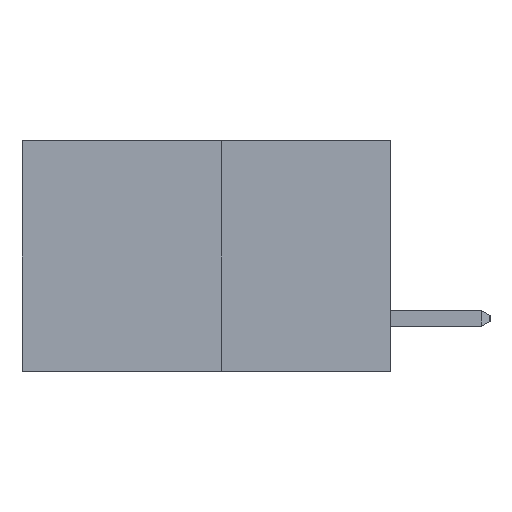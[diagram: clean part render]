
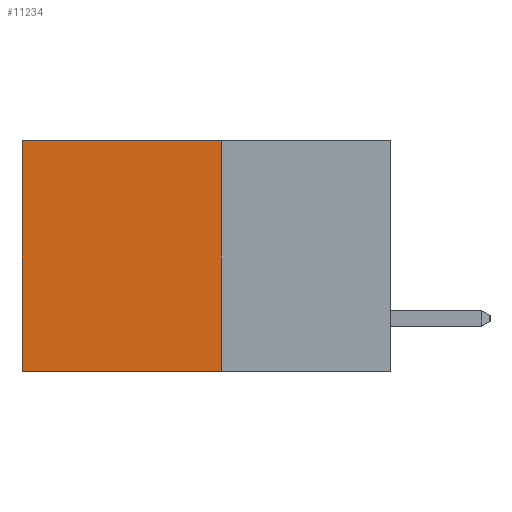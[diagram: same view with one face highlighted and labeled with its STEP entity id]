
A CAD part, left-side view. The second image highlights one B-rep face of the part: STEP entity #11234.
In plain terms, the highlighted planar face has unit normal (-1, 0, 0).
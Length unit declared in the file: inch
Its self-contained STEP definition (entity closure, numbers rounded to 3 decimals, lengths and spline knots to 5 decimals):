
#437 = EDGE_LOOP ( 'NONE', ( #1618, #18572, #18990, #6859 ) ) ;
#762 = DIRECTION ( 'NONE',  ( 0., 0., -1. ) ) ;
#764 = EDGE_CURVE ( 'NONE', #14618, #11002, #4069, .T. ) ;
#1229 = LINE ( 'NONE', #17174, #17666 ) ;
#1618 = ORIENTED_EDGE ( 'NONE', *, *, #764, .T. ) ;
#2950 = VERTEX_POINT ( 'NONE', #10040 ) ;
#3100 = EDGE_CURVE ( 'NONE', #2950, #14618, #7274, .T. ) ;
#3221 = VECTOR ( 'NONE', #16580, 39.37008 ) ;
#4069 = LINE ( 'NONE', #8759, #12252 ) ;
#4211 = AXIS2_PLACEMENT_3D ( 'NONE', #4647, #17748, #7903 ) ;
#4647 = CARTESIAN_POINT ( 'NONE',  ( 0.277, 0.27, -0.37 ) ) ;
#6859 = ORIENTED_EDGE ( 'NONE', *, *, #3100, .T. ) ;
#7274 = LINE ( 'NONE', #12472, #14985 ) ;
#7903 = DIRECTION ( 'NONE',  ( 0., 0., -1. ) ) ;
#8759 = CARTESIAN_POINT ( 'NONE',  ( 0.277, 0.59, -0.37 ) ) ;
#10040 = CARTESIAN_POINT ( 'NONE',  ( 0.277, 0.27, 0. ) ) ;
#11002 = VERTEX_POINT ( 'NONE', #12226 ) ;
#11234 = ADVANCED_FACE ( 'NONE', ( #17237 ), #14452, .F. ) ;
#11778 = CARTESIAN_POINT ( 'NONE',  ( 0.277, 0.59, 0. ) ) ;
#12226 = CARTESIAN_POINT ( 'NONE',  ( 0.277, 0.59, -0.37 ) ) ;
#12252 = VECTOR ( 'NONE', #18794, 39.37008 ) ;
#12472 = CARTESIAN_POINT ( 'NONE',  ( 0.277, 0.27, 0. ) ) ;
#13578 = EDGE_CURVE ( 'NONE', #2950, #15016, #1229, .T. ) ;
#14452 = PLANE ( 'NONE',  #4211 ) ;
#14608 = DIRECTION ( 'NONE',  ( 0., 1., 0. ) ) ;
#14618 = VERTEX_POINT ( 'NONE', #11778 ) ;
#14985 = VECTOR ( 'NONE', #14608, 39.37008 ) ;
#15016 = VERTEX_POINT ( 'NONE', #18363 ) ;
#15093 = EDGE_CURVE ( 'NONE', #15016, #11002, #16318, .T. ) ;
#16318 = LINE ( 'NONE', #18273, #3221 ) ;
#16580 = DIRECTION ( 'NONE',  ( 0., 1., 0. ) ) ;
#17174 = CARTESIAN_POINT ( 'NONE',  ( 0.277, 0.27, -0.37 ) ) ;
#17237 = FACE_OUTER_BOUND ( 'NONE', #437, .T. ) ;
#17666 = VECTOR ( 'NONE', #762, 39.37008 ) ;
#17748 = DIRECTION ( 'NONE',  ( 1., 0., 0. ) ) ;
#18273 = CARTESIAN_POINT ( 'NONE',  ( 0.277, 0.27, -0.37 ) ) ;
#18363 = CARTESIAN_POINT ( 'NONE',  ( 0.277, 0.27, -0.37 ) ) ;
#18572 = ORIENTED_EDGE ( 'NONE', *, *, #15093, .F. ) ;
#18794 = DIRECTION ( 'NONE',  ( 0., 0., -1. ) ) ;
#18990 = ORIENTED_EDGE ( 'NONE', *, *, #13578, .F. ) ;
